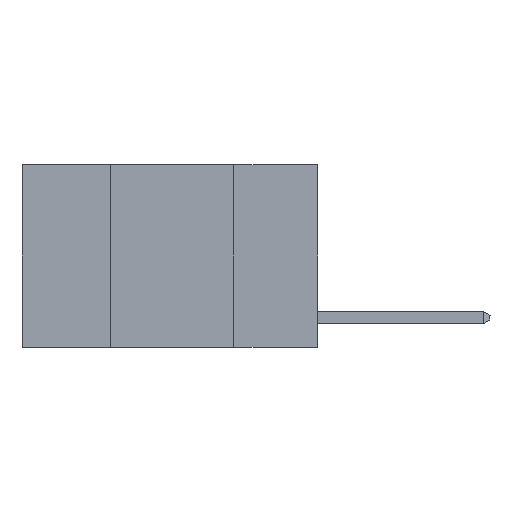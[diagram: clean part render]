
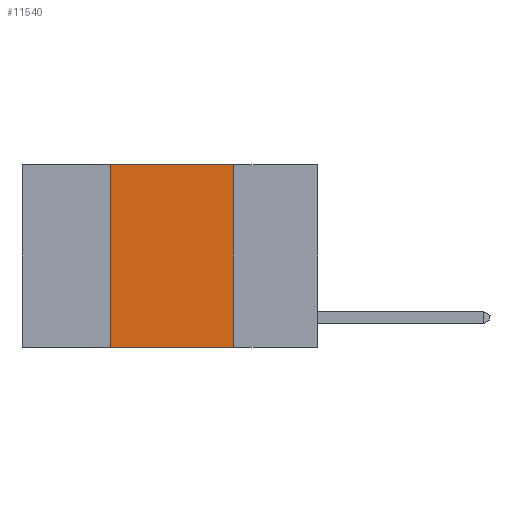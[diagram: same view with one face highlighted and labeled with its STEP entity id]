
A CAD part, left-side view. The second image highlights one B-rep face of the part: STEP entity #11540.
In plain terms, the highlighted planar face has unit normal (-1, 0, 0).
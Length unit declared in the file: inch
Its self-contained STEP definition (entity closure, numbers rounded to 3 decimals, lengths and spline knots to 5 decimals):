
#1015 = EDGE_CURVE ( 'NONE', #10725, #13153, #9500, .T. ) ;
#3139 = VERTEX_POINT ( 'NONE', #4396 ) ;
#3146 = VERTEX_POINT ( 'NONE', #6429 ) ;
#4396 = CARTESIAN_POINT ( 'NONE',  ( 0., 0.42, -0.37 ) ) ;
#6429 = CARTESIAN_POINT ( 'NONE',  ( 0., 0.42, 0. ) ) ;
#6765 = VECTOR ( 'NONE', #14245, 39.37008 ) ;
#7284 = CARTESIAN_POINT ( 'NONE',  ( 0., 0.42, 0. ) ) ;
#7894 = CARTESIAN_POINT ( 'NONE',  ( 0., 0.6, 0. ) ) ;
#9500 = LINE ( 'NONE', #19121, #13521 ) ;
#9543 = CARTESIAN_POINT ( 'NONE',  ( 0., 0.17, 0. ) ) ;
#9775 = ORIENTED_EDGE ( 'NONE', *, *, #1015, .F. ) ;
#9807 = EDGE_CURVE ( 'NONE', #3146, #10725, #22514, .T. ) ;
#9854 = DIRECTION ( 'NONE',  ( 0., 0., -1. ) ) ;
#10019 = LINE ( 'NONE', #21847, #14646 ) ;
#10725 = VERTEX_POINT ( 'NONE', #9543 ) ;
#11540 = ADVANCED_FACE ( 'NONE', ( #22424 ), #15723, .F. ) ;
#11855 = LINE ( 'NONE', #7284, #21746 ) ;
#12284 = CARTESIAN_POINT ( 'NONE',  ( 0., 0.6, 0. ) ) ;
#13153 = VERTEX_POINT ( 'NONE', #22622 ) ;
#13521 = VECTOR ( 'NONE', #19010, 39.37008 ) ;
#14119 = AXIS2_PLACEMENT_3D ( 'NONE', #7894, #21700, #9854 ) ;
#14245 = DIRECTION ( 'NONE',  ( 0., -1., 0. ) ) ;
#14646 = VECTOR ( 'NONE', #23812, 39.37008 ) ;
#15022 = ORIENTED_EDGE ( 'NONE', *, *, #9807, .F. ) ;
#15723 = PLANE ( 'NONE',  #14119 ) ;
#15746 = EDGE_LOOP ( 'NONE', ( #9775, #15022, #25515, #16277 ) ) ;
#16277 = ORIENTED_EDGE ( 'NONE', *, *, #20571, .T. ) ;
#18742 = EDGE_CURVE ( 'NONE', #3139, #3146, #11855, .T. ) ;
#19010 = DIRECTION ( 'NONE',  ( 0., 0., -1. ) ) ;
#19118 = DIRECTION ( 'NONE',  ( 0., 0., 1. ) ) ;
#19121 = CARTESIAN_POINT ( 'NONE',  ( 0., 0.17, 0. ) ) ;
#20571 = EDGE_CURVE ( 'NONE', #3139, #13153, #10019, .T. ) ;
#21700 = DIRECTION ( 'NONE',  ( 1., 0., 0. ) ) ;
#21746 = VECTOR ( 'NONE', #19118, 39.37008 ) ;
#21847 = CARTESIAN_POINT ( 'NONE',  ( 0., 0.6, -0.37 ) ) ;
#22424 = FACE_OUTER_BOUND ( 'NONE', #15746, .T. ) ;
#22514 = LINE ( 'NONE', #12284, #6765 ) ;
#22622 = CARTESIAN_POINT ( 'NONE',  ( 0., 0.17, -0.37 ) ) ;
#23812 = DIRECTION ( 'NONE',  ( 0., -1., 0. ) ) ;
#25515 = ORIENTED_EDGE ( 'NONE', *, *, #18742, .F. ) ;
